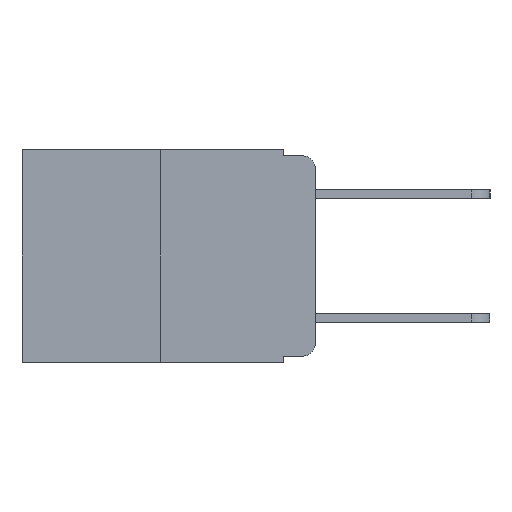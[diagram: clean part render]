
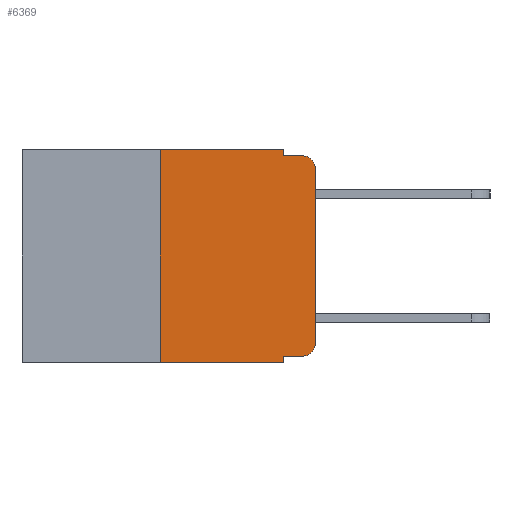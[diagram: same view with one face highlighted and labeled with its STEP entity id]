
A CAD part, left-side view. The second image highlights one B-rep face of the part: STEP entity #6369.
In plain terms, the highlighted planar face has unit normal (-1, 0, 0).
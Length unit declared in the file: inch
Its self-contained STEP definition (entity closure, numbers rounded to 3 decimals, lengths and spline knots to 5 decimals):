
#46 = EDGE_CURVE ( 'NONE', #1211, #21968, #4504, .T. ) ;
#140 = VECTOR ( 'NONE', #2471, 39.37008 ) ;
#274 = CARTESIAN_POINT ( 'NONE',  ( 0., 0.051, -0.333 ) ) ;
#658 = EDGE_CURVE ( 'NONE', #18301, #10068, #1857, .T. ) ;
#1008 = DIRECTION ( 'NONE',  ( 0., -1., 0. ) ) ;
#1211 = VERTEX_POINT ( 'NONE', #21079 ) ;
#1414 = ORIENTED_EDGE ( 'NONE', *, *, #2255, .F. ) ;
#1466 = VERTEX_POINT ( 'NONE', #16344 ) ;
#1857 = LINE ( 'NONE', #9349, #22063 ) ;
#2255 = EDGE_CURVE ( 'NONE', #1466, #1211, #9423, .T. ) ;
#2455 = DIRECTION ( 'NONE',  ( -1., 0., 0. ) ) ;
#2471 = DIRECTION ( 'NONE',  ( 0., 0., -1. ) ) ;
#3169 = ORIENTED_EDGE ( 'NONE', *, *, #22653, .T. ) ;
#3428 = LINE ( 'NONE', #21099, #13956 ) ;
#3561 = DIRECTION ( 'NONE',  ( 0., -1., 0. ) ) ;
#3648 = EDGE_CURVE ( 'NONE', #21968, #18301, #5663, .T. ) ;
#4195 = DIRECTION ( 'NONE',  ( 0., 0., -1. ) ) ;
#4231 = AXIS2_PLACEMENT_3D ( 'NONE', #14356, #2455, #16315 ) ;
#4317 = CARTESIAN_POINT ( 'NONE',  ( 0., 0.02, -0.03 ) ) ;
#4504 = LINE ( 'NONE', #20852, #9215 ) ;
#4890 = LINE ( 'NONE', #21756, #9593 ) ;
#5021 = CIRCLE ( 'NONE', #4231, 0.02 ) ;
#5069 = CARTESIAN_POINT ( 'NONE',  ( 0., 0.051, 0. ) ) ;
#5663 = LINE ( 'NONE', #5069, #140 ) ;
#6342 = DIRECTION ( 'NONE',  ( 0., 0., -1. ) ) ;
#6369 = ADVANCED_FACE ( 'NONE', ( #22123 ), #9276, .F. ) ;
#6950 = EDGE_LOOP ( 'NONE', ( #20809, #17141, #8176, #7146, #12636, #1414, #3169, #9239, #21525, #25004 ) ) ;
#7146 = ORIENTED_EDGE ( 'NONE', *, *, #3648, .F. ) ;
#7312 = VERTEX_POINT ( 'NONE', #13277 ) ;
#7360 = VERTEX_POINT ( 'NONE', #274 ) ;
#8176 = ORIENTED_EDGE ( 'NONE', *, *, #658, .F. ) ;
#9215 = VECTOR ( 'NONE', #14572, 39.37008 ) ;
#9239 = ORIENTED_EDGE ( 'NONE', *, *, #19898, .F. ) ;
#9276 = PLANE ( 'NONE',  #24203 ) ;
#9312 = VERTEX_POINT ( 'NONE', #12651 ) ;
#9349 = CARTESIAN_POINT ( 'NONE',  ( 0., 0.051, -0.01 ) ) ;
#9423 = LINE ( 'NONE', #12693, #12733 ) ;
#9591 = DIRECTION ( 'NONE',  ( 0., 0., -1. ) ) ;
#9593 = VECTOR ( 'NONE', #12248, 39.37008 ) ;
#9892 = CARTESIAN_POINT ( 'NONE',  ( 0., 0.051, -0.01 ) ) ;
#10068 = VERTEX_POINT ( 'NONE', #23306 ) ;
#10183 = EDGE_CURVE ( 'NONE', #9312, #10068, #13792, .T. ) ;
#11539 = CARTESIAN_POINT ( 'NONE',  ( 0., 0.051, -0.333 ) ) ;
#12248 = DIRECTION ( 'NONE',  ( 0., 0., 1. ) ) ;
#12423 = LINE ( 'NONE', #11539, #21403 ) ;
#12636 = ORIENTED_EDGE ( 'NONE', *, *, #46, .F. ) ;
#12651 = CARTESIAN_POINT ( 'NONE',  ( 0., 0., -0.03 ) ) ;
#12693 = CARTESIAN_POINT ( 'NONE',  ( 0., 0.25, 0. ) ) ;
#12733 = VECTOR ( 'NONE', #18537, 39.37008 ) ;
#13277 = CARTESIAN_POINT ( 'NONE',  ( 0., 0.02, -0.333 ) ) ;
#13792 = CIRCLE ( 'NONE', #19695, 0.02 ) ;
#13956 = VECTOR ( 'NONE', #9591, 39.37008 ) ;
#14356 = CARTESIAN_POINT ( 'NONE',  ( 0., 0.02, -0.313 ) ) ;
#14572 = DIRECTION ( 'NONE',  ( 0., -1., 0. ) ) ;
#14783 = LINE ( 'NONE', #20648, #23698 ) ;
#15197 = DIRECTION ( 'NONE',  ( 0., -1., 0. ) ) ;
#16053 = EDGE_CURVE ( 'NONE', #7312, #23218, #5021, .T. ) ;
#16315 = DIRECTION ( 'NONE',  ( 0., 0., -1. ) ) ;
#16344 = CARTESIAN_POINT ( 'NONE',  ( 0., 0.25, -0.343 ) ) ;
#16735 = CARTESIAN_POINT ( 'NONE',  ( 0., 0., -0.313 ) ) ;
#17141 = ORIENTED_EDGE ( 'NONE', *, *, #10183, .T. ) ;
#17346 = EDGE_CURVE ( 'NONE', #7360, #7312, #12423, .T. ) ;
#18024 = DIRECTION ( 'NONE',  ( -1., 0., 0. ) ) ;
#18301 = VERTEX_POINT ( 'NONE', #9892 ) ;
#18537 = DIRECTION ( 'NONE',  ( 0., 0., 1. ) ) ;
#19083 = CARTESIAN_POINT ( 'NONE',  ( 0., 0.051, 0. ) ) ;
#19401 = VERTEX_POINT ( 'NONE', #22826 ) ;
#19695 = AXIS2_PLACEMENT_3D ( 'NONE', #4317, #18024, #6342 ) ;
#19898 = EDGE_CURVE ( 'NONE', #7360, #19401, #3428, .T. ) ;
#20220 = DIRECTION ( 'NONE',  ( 1., 0., 0. ) ) ;
#20648 = CARTESIAN_POINT ( 'NONE',  ( 0., 0.473, -0.343 ) ) ;
#20809 = ORIENTED_EDGE ( 'NONE', *, *, #23025, .T. ) ;
#20852 = CARTESIAN_POINT ( 'NONE',  ( 0., 0.473, 0. ) ) ;
#21079 = CARTESIAN_POINT ( 'NONE',  ( 0., 0.25, 0. ) ) ;
#21099 = CARTESIAN_POINT ( 'NONE',  ( 0., 0.051, 0. ) ) ;
#21403 = VECTOR ( 'NONE', #3561, 39.37008 ) ;
#21525 = ORIENTED_EDGE ( 'NONE', *, *, #17346, .T. ) ;
#21756 = CARTESIAN_POINT ( 'NONE',  ( 0., 0., 0. ) ) ;
#21968 = VERTEX_POINT ( 'NONE', #19083 ) ;
#22063 = VECTOR ( 'NONE', #15197, 39.37008 ) ;
#22123 = FACE_OUTER_BOUND ( 'NONE', #6950, .T. ) ;
#22653 = EDGE_CURVE ( 'NONE', #1466, #19401, #14783, .T. ) ;
#22826 = CARTESIAN_POINT ( 'NONE',  ( 0., 0.051, -0.343 ) ) ;
#23025 = EDGE_CURVE ( 'NONE', #23218, #9312, #4890, .T. ) ;
#23218 = VERTEX_POINT ( 'NONE', #16735 ) ;
#23306 = CARTESIAN_POINT ( 'NONE',  ( 0., 0.02, -0.01 ) ) ;
#23698 = VECTOR ( 'NONE', #1008, 39.37008 ) ;
#24081 = CARTESIAN_POINT ( 'NONE',  ( 0., 0.473, 0. ) ) ;
#24203 = AXIS2_PLACEMENT_3D ( 'NONE', #24081, #20220, #4195 ) ;
#25004 = ORIENTED_EDGE ( 'NONE', *, *, #16053, .T. ) ;
